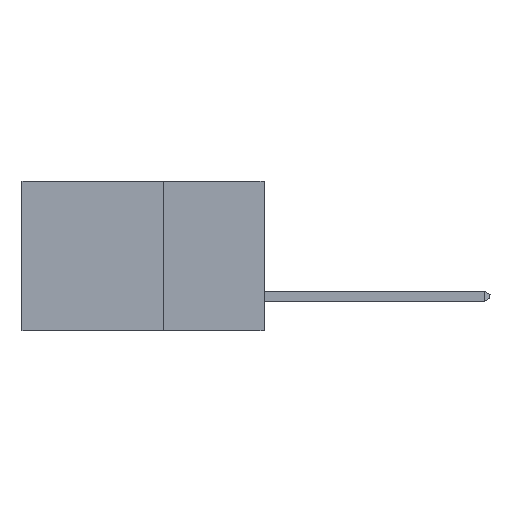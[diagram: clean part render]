
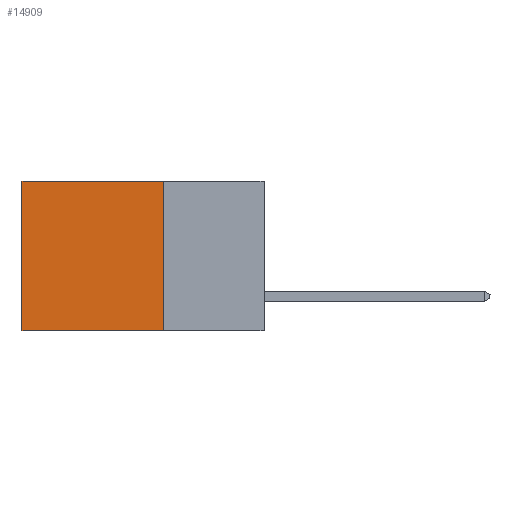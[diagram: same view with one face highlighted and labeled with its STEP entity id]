
A CAD part, left-side view. The second image highlights one B-rep face of the part: STEP entity #14909.
In plain terms, the highlighted planar face has unit normal (-1, 0, 0).
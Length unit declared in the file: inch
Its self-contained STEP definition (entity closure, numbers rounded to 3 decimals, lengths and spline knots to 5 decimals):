
#312 = CARTESIAN_POINT ( 'NONE',  ( 0.298, 0.25, -0.37 ) ) ;
#1083 = VERTEX_POINT ( 'NONE', #312 ) ;
#1197 = CARTESIAN_POINT ( 'NONE',  ( 0.298, 0.25, 0. ) ) ;
#2255 = VERTEX_POINT ( 'NONE', #7124 ) ;
#2865 = CARTESIAN_POINT ( 'NONE',  ( 0.298, 0.25, 0. ) ) ;
#2909 = LINE ( 'NONE', #10612, #7602 ) ;
#4347 = VERTEX_POINT ( 'NONE', #6116 ) ;
#4630 = ORIENTED_EDGE ( 'NONE', *, *, #7154, .T. ) ;
#4848 = VECTOR ( 'NONE', #11577, 39.37008 ) ;
#5913 = EDGE_LOOP ( 'NONE', ( #11681, #10887, #12614, #4630 ) ) ;
#6116 = CARTESIAN_POINT ( 'NONE',  ( 0.298, 0.25, 0. ) ) ;
#6157 = DIRECTION ( 'NONE',  ( 0., 0., -1. ) ) ;
#6557 = EDGE_CURVE ( 'NONE', #1083, #15868, #2909, .T. ) ;
#6671 = CARTESIAN_POINT ( 'NONE',  ( 0.298, 0.6, 0. ) ) ;
#7124 = CARTESIAN_POINT ( 'NONE',  ( 0.298, 0.6, 0. ) ) ;
#7154 = EDGE_CURVE ( 'NONE', #4347, #2255, #9043, .T. ) ;
#7266 = LINE ( 'NONE', #6671, #8618 ) ;
#7505 = LINE ( 'NONE', #9584, #15276 ) ;
#7602 = VECTOR ( 'NONE', #13119, 39.37008 ) ;
#7962 = DIRECTION ( 'NONE',  ( 0., 0., -1. ) ) ;
#8618 = VECTOR ( 'NONE', #7962, 39.37008 ) ;
#9043 = LINE ( 'NONE', #2865, #4848 ) ;
#9584 = CARTESIAN_POINT ( 'NONE',  ( 0.298, 0.25, 0. ) ) ;
#9612 = AXIS2_PLACEMENT_3D ( 'NONE', #1197, #14577, #6157 ) ;
#9993 = EDGE_CURVE ( 'NONE', #2255, #15868, #7266, .T. ) ;
#10443 = CARTESIAN_POINT ( 'NONE',  ( 0.298, 0.6, -0.37 ) ) ;
#10612 = CARTESIAN_POINT ( 'NONE',  ( 0.298, 0.25, -0.37 ) ) ;
#10887 = ORIENTED_EDGE ( 'NONE', *, *, #6557, .F. ) ;
#11128 = PLANE ( 'NONE',  #9612 ) ;
#11422 = DIRECTION ( 'NONE',  ( 0., 0., -1. ) ) ;
#11577 = DIRECTION ( 'NONE',  ( 0., 1., 0. ) ) ;
#11681 = ORIENTED_EDGE ( 'NONE', *, *, #9993, .T. ) ;
#11804 = FACE_OUTER_BOUND ( 'NONE', #5913, .T. ) ;
#12614 = ORIENTED_EDGE ( 'NONE', *, *, #12957, .F. ) ;
#12957 = EDGE_CURVE ( 'NONE', #4347, #1083, #7505, .T. ) ;
#13119 = DIRECTION ( 'NONE',  ( 0., 1., 0. ) ) ;
#14577 = DIRECTION ( 'NONE',  ( 1., 0., 0. ) ) ;
#14909 = ADVANCED_FACE ( 'NONE', ( #11804 ), #11128, .F. ) ;
#15276 = VECTOR ( 'NONE', #11422, 39.37008 ) ;
#15868 = VERTEX_POINT ( 'NONE', #10443 ) ;
